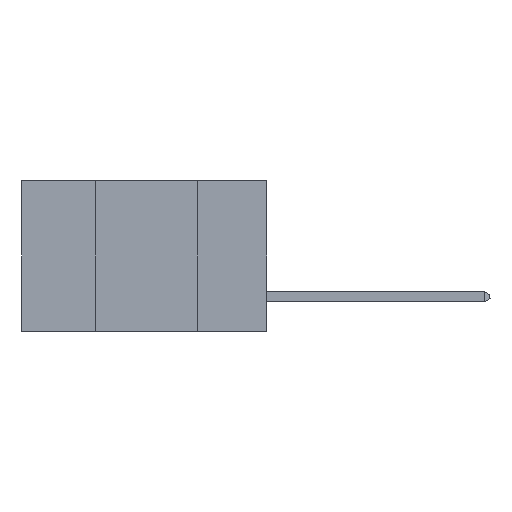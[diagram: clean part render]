
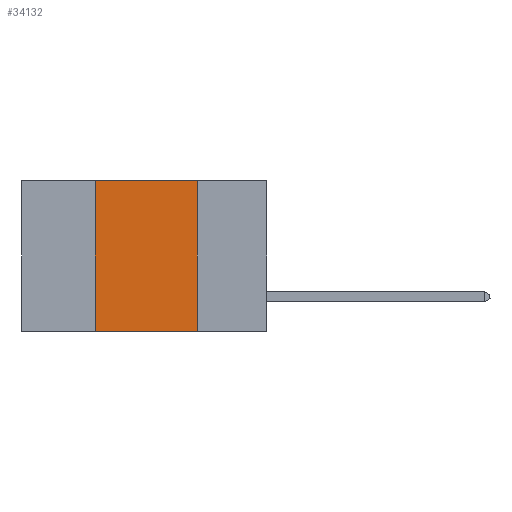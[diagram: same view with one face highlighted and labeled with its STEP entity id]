
A CAD part, left-side view. The second image highlights one B-rep face of the part: STEP entity #34132.
In plain terms, the highlighted planar face has unit normal (-1, 0, 0).
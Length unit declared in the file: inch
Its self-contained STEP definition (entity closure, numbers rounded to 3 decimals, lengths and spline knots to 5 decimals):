
#131 = CARTESIAN_POINT ( 'NONE',  ( 0., 0.6, -0.37 ) ) ;
#482 = EDGE_CURVE ( 'NONE', #34351, #9428, #1928, .T. ) ;
#791 = CARTESIAN_POINT ( 'NONE',  ( 0., 0.42, -0.37 ) ) ;
#1881 = CARTESIAN_POINT ( 'NONE',  ( 0., 0.42, 0. ) ) ;
#1928 = LINE ( 'NONE', #34325, #32222 ) ;
#2624 = VECTOR ( 'NONE', #28159, 39.37008 ) ;
#2789 = DIRECTION ( 'NONE',  ( 0., 0., -1. ) ) ;
#3158 = CARTESIAN_POINT ( 'NONE',  ( 0., 0.17, -0.37 ) ) ;
#5044 = LINE ( 'NONE', #131, #37229 ) ;
#5638 = DIRECTION ( 'NONE',  ( 0., -1., 0. ) ) ;
#7667 = ORIENTED_EDGE ( 'NONE', *, *, #38176, .T. ) ;
#9428 = VERTEX_POINT ( 'NONE', #1881 ) ;
#10388 = ORIENTED_EDGE ( 'NONE', *, *, #37578, .F. ) ;
#12775 = CARTESIAN_POINT ( 'NONE',  ( 0., 0.17, 0. ) ) ;
#12920 = EDGE_LOOP ( 'NONE', ( #10388, #17154, #16955, #7667 ) ) ;
#13246 = FACE_OUTER_BOUND ( 'NONE', #12920, .T. ) ;
#14249 = EDGE_CURVE ( 'NONE', #9428, #20232, #35830, .T. ) ;
#15388 = PLANE ( 'NONE',  #28099 ) ;
#15869 = VECTOR ( 'NONE', #5638, 39.37008 ) ;
#16955 = ORIENTED_EDGE ( 'NONE', *, *, #482, .F. ) ;
#17154 = ORIENTED_EDGE ( 'NONE', *, *, #14249, .F. ) ;
#20232 = VERTEX_POINT ( 'NONE', #12775 ) ;
#25169 = CARTESIAN_POINT ( 'NONE',  ( 0., 0.17, 0. ) ) ;
#26141 = LINE ( 'NONE', #25169, #2624 ) ;
#27671 = CARTESIAN_POINT ( 'NONE',  ( 0., 0.6, 0. ) ) ;
#28099 = AXIS2_PLACEMENT_3D ( 'NONE', #27671, #40426, #2789 ) ;
#28159 = DIRECTION ( 'NONE',  ( 0., 0., -1. ) ) ;
#28210 = DIRECTION ( 'NONE',  ( 0., 0., 1. ) ) ;
#32222 = VECTOR ( 'NONE', #28210, 39.37008 ) ;
#34132 = ADVANCED_FACE ( 'NONE', ( #13246 ), #15388, .F. ) ;
#34325 = CARTESIAN_POINT ( 'NONE',  ( 0., 0.42, 0. ) ) ;
#34351 = VERTEX_POINT ( 'NONE', #791 ) ;
#35693 = VERTEX_POINT ( 'NONE', #3158 ) ;
#35830 = LINE ( 'NONE', #39570, #15869 ) ;
#37229 = VECTOR ( 'NONE', #37627, 39.37008 ) ;
#37578 = EDGE_CURVE ( 'NONE', #20232, #35693, #26141, .T. ) ;
#37627 = DIRECTION ( 'NONE',  ( 0., -1., 0. ) ) ;
#38176 = EDGE_CURVE ( 'NONE', #34351, #35693, #5044, .T. ) ;
#39570 = CARTESIAN_POINT ( 'NONE',  ( 0., 0.6, 0. ) ) ;
#40426 = DIRECTION ( 'NONE',  ( 1., 0., 0. ) ) ;
